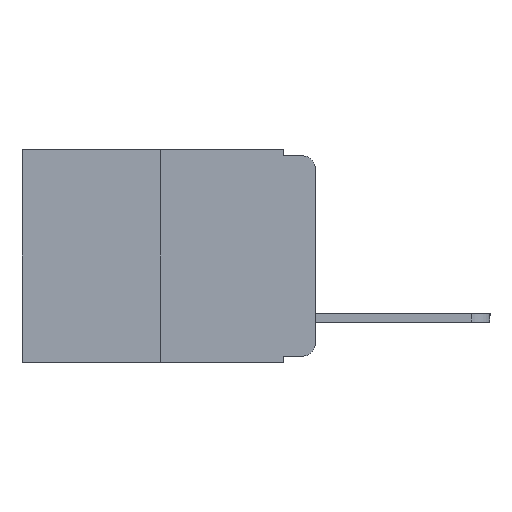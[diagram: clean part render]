
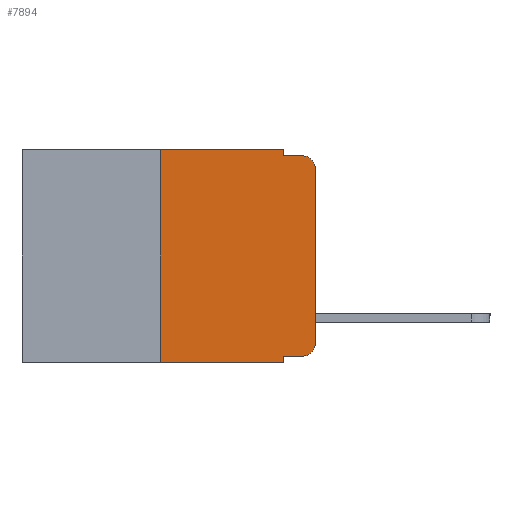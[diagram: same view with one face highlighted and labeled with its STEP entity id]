
A CAD part, left-side view. The second image highlights one B-rep face of the part: STEP entity #7894.
In plain terms, the highlighted planar face has unit normal (-1, 0, 0).
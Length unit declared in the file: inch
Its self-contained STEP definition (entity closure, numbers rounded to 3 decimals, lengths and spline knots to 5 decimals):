
#140 = VECTOR ( 'NONE', #12407, 39.37008 ) ;
#862 = CARTESIAN_POINT ( 'NONE',  ( 0., 0.25, -0.343 ) ) ;
#1083 = DIRECTION ( 'NONE',  ( 0., 0., 1. ) ) ;
#1193 = PLANE ( 'NONE',  #19518 ) ;
#1270 = LINE ( 'NONE', #21830, #140 ) ;
#1497 = CARTESIAN_POINT ( 'NONE',  ( 0., 0., 0. ) ) ;
#1785 = ORIENTED_EDGE ( 'NONE', *, *, #3853, .F. ) ;
#2891 = DIRECTION ( 'NONE',  ( 0., -1., 0. ) ) ;
#3015 = CARTESIAN_POINT ( 'NONE',  ( 0., 0.02, -0.333 ) ) ;
#3077 = VERTEX_POINT ( 'NONE', #18896 ) ;
#3410 = VERTEX_POINT ( 'NONE', #12786 ) ;
#3563 = VECTOR ( 'NONE', #2891, 39.37008 ) ;
#3625 = VERTEX_POINT ( 'NONE', #862 ) ;
#3853 = EDGE_CURVE ( 'NONE', #10495, #14817, #1270, .T. ) ;
#4065 = EDGE_CURVE ( 'NONE', #3625, #3077, #18144, .T. ) ;
#4191 = ORIENTED_EDGE ( 'NONE', *, *, #15718, .F. ) ;
#4374 = CARTESIAN_POINT ( 'NONE',  ( 0., 0.473, 0. ) ) ;
#4522 = DIRECTION ( 'NONE',  ( 0., 0., -1. ) ) ;
#4657 = ORIENTED_EDGE ( 'NONE', *, *, #15298, .T. ) ;
#4730 = VERTEX_POINT ( 'NONE', #16041 ) ;
#4795 = CARTESIAN_POINT ( 'NONE',  ( 0., 0.473, 0. ) ) ;
#4979 = VERTEX_POINT ( 'NONE', #13858 ) ;
#5484 = EDGE_CURVE ( 'NONE', #3625, #8619, #10449, .T. ) ;
#5625 = VECTOR ( 'NONE', #12295, 39.37008 ) ;
#5952 = ORIENTED_EDGE ( 'NONE', *, *, #17605, .T. ) ;
#6184 = CIRCLE ( 'NONE', #17903, 0.02 ) ;
#6864 = VECTOR ( 'NONE', #19687, 39.37008 ) ;
#7152 = VERTEX_POINT ( 'NONE', #16264 ) ;
#7188 = DIRECTION ( 'NONE',  ( 0., -1., 0. ) ) ;
#7464 = CARTESIAN_POINT ( 'NONE',  ( 0., 0.02, -0.03 ) ) ;
#7894 = ADVANCED_FACE ( 'NONE', ( #22080 ), #1193, .F. ) ;
#8194 = EDGE_CURVE ( 'NONE', #21433, #4730, #16211, .T. ) ;
#8222 = VECTOR ( 'NONE', #19796, 39.37008 ) ;
#8386 = DIRECTION ( 'NONE',  ( 0., 0., 1. ) ) ;
#8397 = CARTESIAN_POINT ( 'NONE',  ( 0., 0.473, -0.343 ) ) ;
#8619 = VERTEX_POINT ( 'NONE', #19735 ) ;
#8679 = LINE ( 'NONE', #1497, #13688 ) ;
#9160 = DIRECTION ( 'NONE',  ( 0., 0., -1. ) ) ;
#9459 = CARTESIAN_POINT ( 'NONE',  ( 0., 0.051, -0.333 ) ) ;
#9493 = ORIENTED_EDGE ( 'NONE', *, *, #11562, .T. ) ;
#9576 = CARTESIAN_POINT ( 'NONE',  ( 0., 0.051, 0. ) ) ;
#10121 = VECTOR ( 'NONE', #7188, 39.37008 ) ;
#10449 = LINE ( 'NONE', #17568, #14992 ) ;
#10486 = EDGE_CURVE ( 'NONE', #8619, #4979, #12625, .T. ) ;
#10495 = VERTEX_POINT ( 'NONE', #16726 ) ;
#11230 = CARTESIAN_POINT ( 'NONE',  ( 0., 0.02, -0.01 ) ) ;
#11562 = EDGE_CURVE ( 'NONE', #7152, #21433, #15891, .T. ) ;
#12295 = DIRECTION ( 'NONE',  ( 0., 0., -1. ) ) ;
#12407 = DIRECTION ( 'NONE',  ( 0., -1., 0. ) ) ;
#12625 = LINE ( 'NONE', #4795, #3563 ) ;
#12663 = ORIENTED_EDGE ( 'NONE', *, *, #4065, .T. ) ;
#12681 = LINE ( 'NONE', #9576, #8222 ) ;
#12786 = CARTESIAN_POINT ( 'NONE',  ( 0., 0., -0.03 ) ) ;
#13688 = VECTOR ( 'NONE', #8386, 39.37008 ) ;
#13858 = CARTESIAN_POINT ( 'NONE',  ( 0., 0.051, 0. ) ) ;
#14360 = DIRECTION ( 'NONE',  ( 0., 0., -1. ) ) ;
#14720 = DIRECTION ( 'NONE',  ( 1., 0., 0. ) ) ;
#14817 = VERTEX_POINT ( 'NONE', #11230 ) ;
#14848 = EDGE_LOOP ( 'NONE', ( #5952, #4657, #1785, #4191, #17233, #19381, #12663, #21164, #9493, #19296 ) ) ;
#14992 = VECTOR ( 'NONE', #1083, 39.37008 ) ;
#15188 = LINE ( 'NONE', #20852, #5625 ) ;
#15298 = EDGE_CURVE ( 'NONE', #3410, #14817, #6184, .T. ) ;
#15615 = AXIS2_PLACEMENT_3D ( 'NONE', #17848, #18536, #14360 ) ;
#15718 = EDGE_CURVE ( 'NONE', #4979, #10495, #15188, .T. ) ;
#15891 = LINE ( 'NONE', #9459, #6864 ) ;
#16041 = CARTESIAN_POINT ( 'NONE',  ( 0., 0., -0.313 ) ) ;
#16211 = CIRCLE ( 'NONE', #15615, 0.02 ) ;
#16264 = CARTESIAN_POINT ( 'NONE',  ( 0., 0.051, -0.333 ) ) ;
#16726 = CARTESIAN_POINT ( 'NONE',  ( 0., 0.051, -0.01 ) ) ;
#17233 = ORIENTED_EDGE ( 'NONE', *, *, #10486, .F. ) ;
#17313 = EDGE_CURVE ( 'NONE', #7152, #3077, #12681, .T. ) ;
#17568 = CARTESIAN_POINT ( 'NONE',  ( 0., 0.25, 0. ) ) ;
#17605 = EDGE_CURVE ( 'NONE', #4730, #3410, #8679, .T. ) ;
#17848 = CARTESIAN_POINT ( 'NONE',  ( 0., 0.02, -0.313 ) ) ;
#17903 = AXIS2_PLACEMENT_3D ( 'NONE', #7464, #19383, #9160 ) ;
#18144 = LINE ( 'NONE', #8397, #10121 ) ;
#18536 = DIRECTION ( 'NONE',  ( -1., 0., 0. ) ) ;
#18896 = CARTESIAN_POINT ( 'NONE',  ( 0., 0.051, -0.343 ) ) ;
#19296 = ORIENTED_EDGE ( 'NONE', *, *, #8194, .T. ) ;
#19381 = ORIENTED_EDGE ( 'NONE', *, *, #5484, .F. ) ;
#19383 = DIRECTION ( 'NONE',  ( -1., 0., 0. ) ) ;
#19518 = AXIS2_PLACEMENT_3D ( 'NONE', #4374, #14720, #4522 ) ;
#19687 = DIRECTION ( 'NONE',  ( 0., -1., 0. ) ) ;
#19735 = CARTESIAN_POINT ( 'NONE',  ( 0., 0.25, 0. ) ) ;
#19796 = DIRECTION ( 'NONE',  ( 0., 0., -1. ) ) ;
#20852 = CARTESIAN_POINT ( 'NONE',  ( 0., 0.051, 0. ) ) ;
#21164 = ORIENTED_EDGE ( 'NONE', *, *, #17313, .F. ) ;
#21433 = VERTEX_POINT ( 'NONE', #3015 ) ;
#21830 = CARTESIAN_POINT ( 'NONE',  ( 0., 0.051, -0.01 ) ) ;
#22080 = FACE_OUTER_BOUND ( 'NONE', #14848, .T. ) ;
